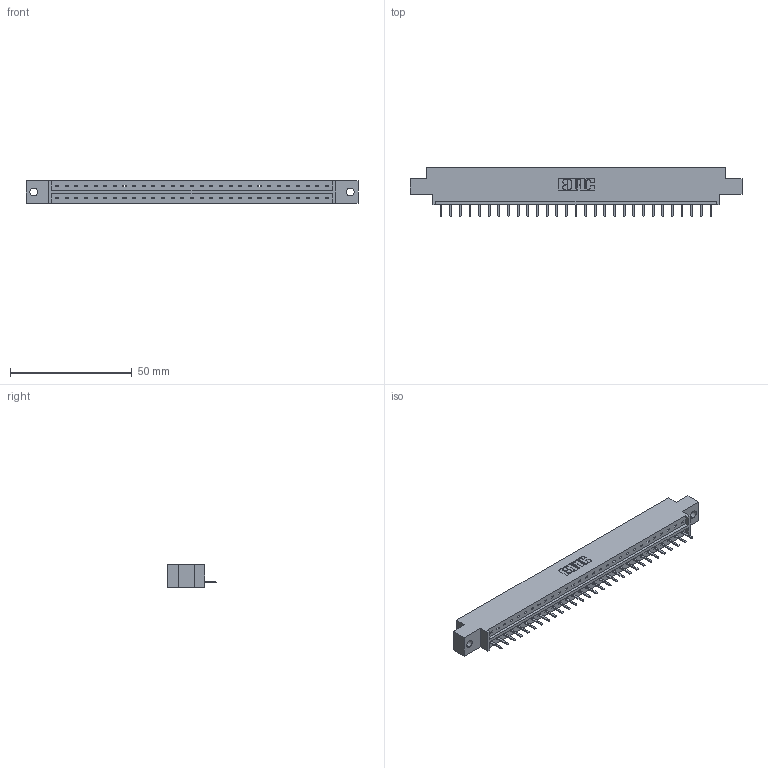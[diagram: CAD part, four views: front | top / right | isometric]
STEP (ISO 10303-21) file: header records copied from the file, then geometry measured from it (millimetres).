
FILE_DESCRIPTION (( 'STEP AP203' ), '1' );
FILE_NAME ('333-029-520-602.STEP', '2018-08-02T16:12:30', ( '' ), ( '' ), 'SwSTEP 2.0', 'SolidWorks 2016', '' );
FILE_SCHEMA (( 'CONFIG_CONTROL_DESIGN' ));
Length unit declared in the file: inch
Products named in the file (3): 333 Part_Offset - .128 Dia; 345-292-001_345-293-120; 333-029-520-602
Assembly tree (30 placements, depth 2):
  333-029-520-602
    333 Part_Offset - .128 Dia
    345-292-001_345-293-120  x29
Bounding box: 136.45 x 20.02 x 9.4 mm (x, y, z)
Volume: 13270.9 mm3; surface area: 13906.9 mm2
Topology: 30 solids, 30 shells, 1916 faces, 5659 edges, 3694 vertices
Faces by surface type: plane 1350, cylinder 566
Entity records: 19659 total; most frequent: CARTESIAN_POINT 3413, ORIENTED_EDGE 3366, DIRECTION 2893, EDGE_CURVE 1683, VECTOR 1551, LINE 1551, VERTEX_POINT 1118, AXIS2_PLACEMENT_3D 671
